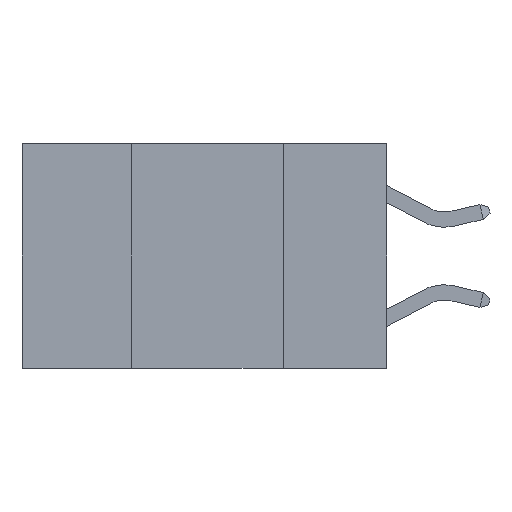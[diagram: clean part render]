
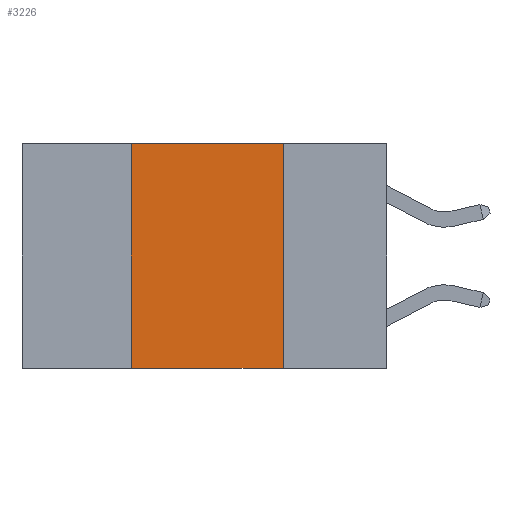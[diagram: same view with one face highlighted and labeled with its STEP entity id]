
A CAD part, left-side view. The second image highlights one B-rep face of the part: STEP entity #3226.
In plain terms, the highlighted planar face has unit normal (-1, 0, 0).
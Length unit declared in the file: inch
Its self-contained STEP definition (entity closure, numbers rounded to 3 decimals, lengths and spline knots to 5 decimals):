
#326 = CARTESIAN_POINT ( 'NONE',  ( 0., 0.6, -0.37 ) ) ;
#610 = CARTESIAN_POINT ( 'NONE',  ( 0., 0.42, 0. ) ) ;
#1793 = DIRECTION ( 'NONE',  ( 1., 0., 0. ) ) ;
#2403 = FACE_OUTER_BOUND ( 'NONE', #9253, .T. ) ;
#2880 = ORIENTED_EDGE ( 'NONE', *, *, #7309, .T. ) ;
#2885 = LINE ( 'NONE', #5104, #4645 ) ;
#3152 = LINE ( 'NONE', #326, #8434 ) ;
#3226 = ADVANCED_FACE ( 'NONE', ( #2403 ), #4849, .F. ) ;
#3294 = CARTESIAN_POINT ( 'NONE',  ( 0., 0.17, 0. ) ) ;
#3369 = CARTESIAN_POINT ( 'NONE',  ( 0., 0.17, -0.37 ) ) ;
#3616 = DIRECTION ( 'NONE',  ( 0., 0., -1. ) ) ;
#3640 = VECTOR ( 'NONE', #8456, 39.37008 ) ;
#3705 = DIRECTION ( 'NONE',  ( 0., 0., 1. ) ) ;
#4326 = CARTESIAN_POINT ( 'NONE',  ( 0., 0.17, 0. ) ) ;
#4378 = VERTEX_POINT ( 'NONE', #610 ) ;
#4447 = DIRECTION ( 'NONE',  ( 0., -1., 0. ) ) ;
#4494 = ORIENTED_EDGE ( 'NONE', *, *, #5843, .F. ) ;
#4645 = VECTOR ( 'NONE', #3705, 39.37008 ) ;
#4849 = PLANE ( 'NONE',  #7335 ) ;
#5072 = VECTOR ( 'NONE', #3616, 39.37008 ) ;
#5104 = CARTESIAN_POINT ( 'NONE',  ( 0., 0.42, 0. ) ) ;
#5843 = EDGE_CURVE ( 'NONE', #4378, #8185, #9048, .T. ) ;
#6208 = ORIENTED_EDGE ( 'NONE', *, *, #7285, .F. ) ;
#6218 = CARTESIAN_POINT ( 'NONE',  ( 0., 0.6, 0. ) ) ;
#6352 = VERTEX_POINT ( 'NONE', #7432 ) ;
#6560 = VERTEX_POINT ( 'NONE', #3369 ) ;
#6924 = LINE ( 'NONE', #4326, #5072 ) ;
#6933 = DIRECTION ( 'NONE',  ( 0., 0., -1. ) ) ;
#6964 = ORIENTED_EDGE ( 'NONE', *, *, #7109, .F. ) ;
#7109 = EDGE_CURVE ( 'NONE', #8185, #6560, #6924, .T. ) ;
#7196 = CARTESIAN_POINT ( 'NONE',  ( 0., 0.6, 0. ) ) ;
#7285 = EDGE_CURVE ( 'NONE', #6352, #4378, #2885, .T. ) ;
#7309 = EDGE_CURVE ( 'NONE', #6352, #6560, #3152, .T. ) ;
#7335 = AXIS2_PLACEMENT_3D ( 'NONE', #6218, #1793, #6933 ) ;
#7432 = CARTESIAN_POINT ( 'NONE',  ( 0., 0.42, -0.37 ) ) ;
#8185 = VERTEX_POINT ( 'NONE', #3294 ) ;
#8434 = VECTOR ( 'NONE', #4447, 39.37008 ) ;
#8456 = DIRECTION ( 'NONE',  ( 0., -1., 0. ) ) ;
#9048 = LINE ( 'NONE', #7196, #3640 ) ;
#9253 = EDGE_LOOP ( 'NONE', ( #6964, #4494, #6208, #2880 ) ) ;
